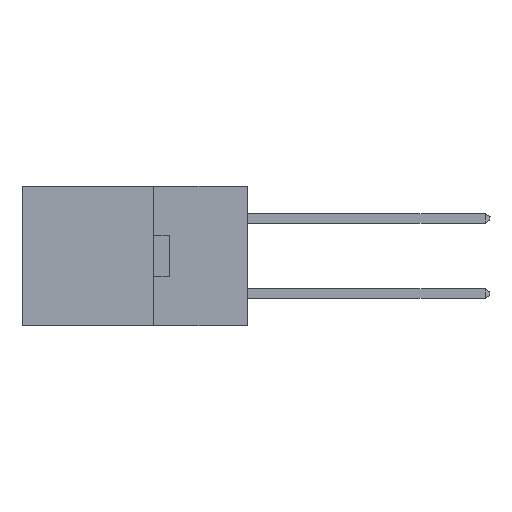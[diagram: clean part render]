
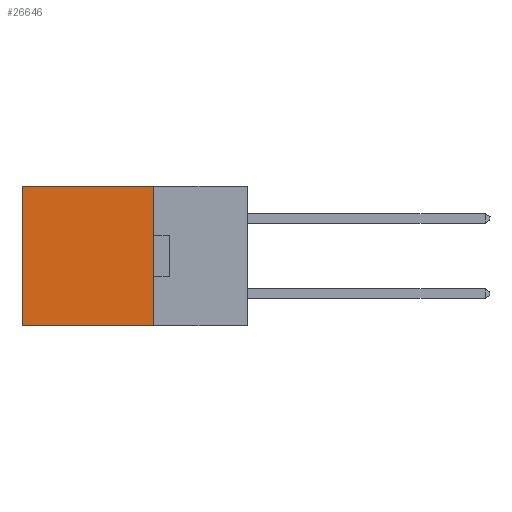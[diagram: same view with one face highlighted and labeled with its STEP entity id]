
A CAD part, left-side view. The second image highlights one B-rep face of the part: STEP entity #26646.
In plain terms, the highlighted planar face has unit normal (-1, 0, 0).
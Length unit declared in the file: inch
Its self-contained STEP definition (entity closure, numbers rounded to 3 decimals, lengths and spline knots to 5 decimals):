
#1807 = ORIENTED_EDGE ( 'NONE', *, *, #16030, .T. ) ;
#2626 = DIRECTION ( 'NONE',  ( 0., 1., 0. ) ) ;
#2847 = LINE ( 'NONE', #11176, #18528 ) ;
#3810 = AXIS2_PLACEMENT_3D ( 'NONE', #23192, #27693, #23627 ) ;
#5861 = EDGE_LOOP ( 'NONE', ( #1807, #13837, #10256, #19723 ) ) ;
#6757 = VECTOR ( 'NONE', #9072, 39.37008 ) ;
#7003 = EDGE_CURVE ( 'NONE', #8341, #7600, #2847, .T. ) ;
#7600 = VERTEX_POINT ( 'NONE', #21326 ) ;
#8341 = VERTEX_POINT ( 'NONE', #24752 ) ;
#9030 = LINE ( 'NONE', #22315, #27999 ) ;
#9072 = DIRECTION ( 'NONE',  ( 0., 0., -1. ) ) ;
#9973 = EDGE_CURVE ( 'NONE', #8341, #25832, #9030, .T. ) ;
#10256 = ORIENTED_EDGE ( 'NONE', *, *, #7003, .F. ) ;
#10472 = CARTESIAN_POINT ( 'NONE',  ( 0.2615, 0.6, 0. ) ) ;
#11176 = CARTESIAN_POINT ( 'NONE',  ( 0.2615, 0.25, -0.37 ) ) ;
#12782 = DIRECTION ( 'NONE',  ( 0., 1., 0. ) ) ;
#13219 = LINE ( 'NONE', #21664, #26392 ) ;
#13837 = ORIENTED_EDGE ( 'NONE', *, *, #20949, .F. ) ;
#14309 = PLANE ( 'NONE',  #3810 ) ;
#15776 = LINE ( 'NONE', #26567, #6757 ) ;
#15810 = DIRECTION ( 'NONE',  ( 0., 0., -1. ) ) ;
#16030 = EDGE_CURVE ( 'NONE', #25832, #24264, #15776, .T. ) ;
#18528 = VECTOR ( 'NONE', #15810, 39.37008 ) ;
#19723 = ORIENTED_EDGE ( 'NONE', *, *, #9973, .T. ) ;
#20949 = EDGE_CURVE ( 'NONE', #7600, #24264, #13219, .T. ) ;
#21326 = CARTESIAN_POINT ( 'NONE',  ( 0.2615, 0.25, -0.37 ) ) ;
#21664 = CARTESIAN_POINT ( 'NONE',  ( 0.2615, 0.25, -0.37 ) ) ;
#22315 = CARTESIAN_POINT ( 'NONE',  ( 0.2615, 0.25, 0. ) ) ;
#23192 = CARTESIAN_POINT ( 'NONE',  ( 0.2615, 0.25, -0.37 ) ) ;
#23627 = DIRECTION ( 'NONE',  ( 0., 0., -1. ) ) ;
#24264 = VERTEX_POINT ( 'NONE', #24274 ) ;
#24274 = CARTESIAN_POINT ( 'NONE',  ( 0.2615, 0.6, -0.37 ) ) ;
#24752 = CARTESIAN_POINT ( 'NONE',  ( 0.2615, 0.25, 0. ) ) ;
#25832 = VERTEX_POINT ( 'NONE', #10472 ) ;
#26093 = FACE_OUTER_BOUND ( 'NONE', #5861, .T. ) ;
#26392 = VECTOR ( 'NONE', #12782, 39.37008 ) ;
#26567 = CARTESIAN_POINT ( 'NONE',  ( 0.2615, 0.6, -0.37 ) ) ;
#26646 = ADVANCED_FACE ( 'NONE', ( #26093 ), #14309, .F. ) ;
#27693 = DIRECTION ( 'NONE',  ( 1., 0., 0. ) ) ;
#27999 = VECTOR ( 'NONE', #2626, 39.37008 ) ;
